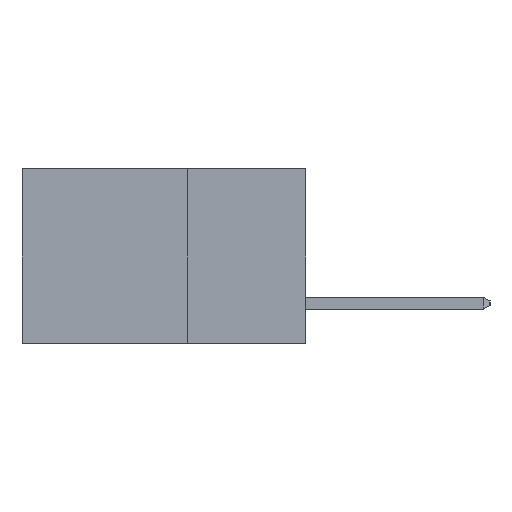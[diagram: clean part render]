
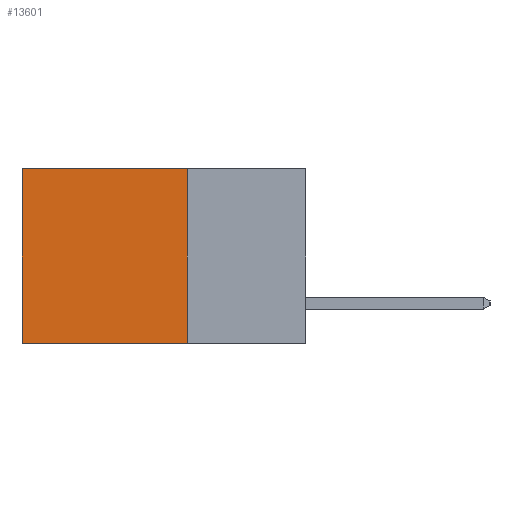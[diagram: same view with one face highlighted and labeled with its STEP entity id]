
A CAD part, left-side view. The second image highlights one B-rep face of the part: STEP entity #13601.
In plain terms, the highlighted planar face has unit normal (-1, 0, 0).
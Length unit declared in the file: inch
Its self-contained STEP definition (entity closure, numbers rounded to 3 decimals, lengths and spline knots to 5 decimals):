
#934 = VERTEX_POINT ( 'NONE', #16081 ) ;
#1545 = VERTEX_POINT ( 'NONE', #6019 ) ;
#2615 = VECTOR ( 'NONE', #13441, 39.37008 ) ;
#3371 = CARTESIAN_POINT ( 'NONE',  ( 0.2615, 0.25, -0.37 ) ) ;
#3599 = CARTESIAN_POINT ( 'NONE',  ( 0.2615, 0.6, -0.37 ) ) ;
#3811 = LINE ( 'NONE', #14386, #12480 ) ;
#3999 = EDGE_LOOP ( 'NONE', ( #14570, #15862, #6145, #9017 ) ) ;
#4687 = EDGE_CURVE ( 'NONE', #1545, #19623, #11838, .T. ) ;
#4903 = CARTESIAN_POINT ( 'NONE',  ( 0.2615, 0.25, -0.37 ) ) ;
#6019 = CARTESIAN_POINT ( 'NONE',  ( 0.2615, 0.6, 0. ) ) ;
#6145 = ORIENTED_EDGE ( 'NONE', *, *, #18116, .F. ) ;
#6919 = DIRECTION ( 'NONE',  ( 0., 0., -1. ) ) ;
#8203 = VECTOR ( 'NONE', #14800, 39.37008 ) ;
#8366 = EDGE_CURVE ( 'NONE', #12385, #19623, #3811, .T. ) ;
#8766 = LINE ( 'NONE', #18128, #8203 ) ;
#9017 = ORIENTED_EDGE ( 'NONE', *, *, #10994, .T. ) ;
#10994 = EDGE_CURVE ( 'NONE', #934, #1545, #21934, .T. ) ;
#11838 = LINE ( 'NONE', #14364, #2615 ) ;
#12286 = AXIS2_PLACEMENT_3D ( 'NONE', #3371, #17200, #6919 ) ;
#12385 = VERTEX_POINT ( 'NONE', #4903 ) ;
#12480 = VECTOR ( 'NONE', #14284, 39.37008 ) ;
#13441 = DIRECTION ( 'NONE',  ( 0., 0., -1. ) ) ;
#13601 = ADVANCED_FACE ( 'NONE', ( #17912 ), #13813, .F. ) ;
#13813 = PLANE ( 'NONE',  #12286 ) ;
#14284 = DIRECTION ( 'NONE',  ( 0., 1., 0. ) ) ;
#14364 = CARTESIAN_POINT ( 'NONE',  ( 0.2615, 0.6, -0.37 ) ) ;
#14386 = CARTESIAN_POINT ( 'NONE',  ( 0.2615, 0.25, -0.37 ) ) ;
#14570 = ORIENTED_EDGE ( 'NONE', *, *, #4687, .T. ) ;
#14800 = DIRECTION ( 'NONE',  ( 0., 0., -1. ) ) ;
#15110 = CARTESIAN_POINT ( 'NONE',  ( 0.2615, 0.25, 0. ) ) ;
#15862 = ORIENTED_EDGE ( 'NONE', *, *, #8366, .F. ) ;
#16081 = CARTESIAN_POINT ( 'NONE',  ( 0.2615, 0.25, 0. ) ) ;
#17200 = DIRECTION ( 'NONE',  ( 1., 0., 0. ) ) ;
#17498 = VECTOR ( 'NONE', #18490, 39.37008 ) ;
#17912 = FACE_OUTER_BOUND ( 'NONE', #3999, .T. ) ;
#18116 = EDGE_CURVE ( 'NONE', #934, #12385, #8766, .T. ) ;
#18128 = CARTESIAN_POINT ( 'NONE',  ( 0.2615, 0.25, -0.37 ) ) ;
#18490 = DIRECTION ( 'NONE',  ( 0., 1., 0. ) ) ;
#19623 = VERTEX_POINT ( 'NONE', #3599 ) ;
#21934 = LINE ( 'NONE', #15110, #17498 ) ;
